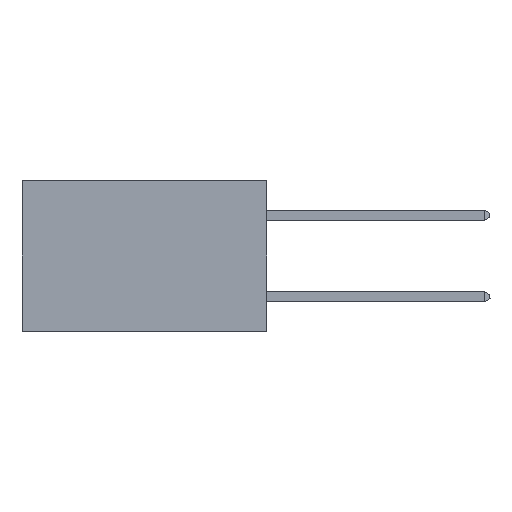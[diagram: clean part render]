
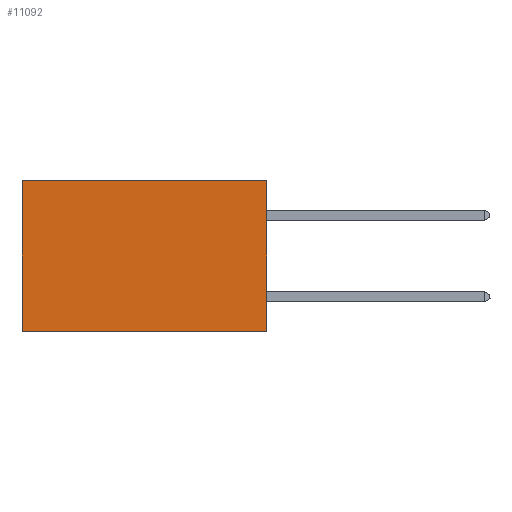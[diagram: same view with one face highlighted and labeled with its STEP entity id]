
A CAD part, left-side view. The second image highlights one B-rep face of the part: STEP entity #11092.
In plain terms, the highlighted planar face has unit normal (-1, 0, 0).
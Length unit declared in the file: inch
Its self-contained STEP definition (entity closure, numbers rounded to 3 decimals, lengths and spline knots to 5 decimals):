
#454 = AXIS2_PLACEMENT_3D ( 'NONE', #13545, #6897, #18457 ) ;
#1673 = ORIENTED_EDGE ( 'NONE', *, *, #16021, .F. ) ;
#1769 = ORIENTED_EDGE ( 'NONE', *, *, #9709, .F. ) ;
#2898 = LINE ( 'NONE', #5772, #15723 ) ;
#3300 = DIRECTION ( 'NONE',  ( 0., 0., -1. ) ) ;
#3677 = VECTOR ( 'NONE', #7392, 39.37008 ) ;
#3735 = EDGE_CURVE ( 'NONE', #11510, #10776, #2898, .T. ) ;
#4346 = EDGE_CURVE ( 'NONE', #15177, #11510, #18508, .T. ) ;
#4684 = CARTESIAN_POINT ( 'NONE',  ( 0.2875, 0., 0. ) ) ;
#5166 = PLANE ( 'NONE',  #454 ) ;
#5332 = VECTOR ( 'NONE', #5885, 39.37008 ) ;
#5772 = CARTESIAN_POINT ( 'NONE',  ( 0.2875, 0.6, 0. ) ) ;
#5885 = DIRECTION ( 'NONE',  ( 0., 1., 0. ) ) ;
#6267 = CARTESIAN_POINT ( 'NONE',  ( 0.2875, 0.6, 0. ) ) ;
#6675 = LINE ( 'NONE', #13383, #15516 ) ;
#6897 = DIRECTION ( 'NONE',  ( 1., 0., 0. ) ) ;
#7115 = ORIENTED_EDGE ( 'NONE', *, *, #3735, .T. ) ;
#7392 = DIRECTION ( 'NONE',  ( 0., 1., 0. ) ) ;
#7498 = DIRECTION ( 'NONE',  ( 0., 0., -1. ) ) ;
#9268 = CARTESIAN_POINT ( 'NONE',  ( 0.2875, 0., -0.37 ) ) ;
#9709 = EDGE_CURVE ( 'NONE', #15177, #10811, #6675, .T. ) ;
#10734 = CARTESIAN_POINT ( 'NONE',  ( 0.2875, 0., 0. ) ) ;
#10776 = VERTEX_POINT ( 'NONE', #12766 ) ;
#10811 = VERTEX_POINT ( 'NONE', #12911 ) ;
#11092 = ADVANCED_FACE ( 'NONE', ( #17744 ), #5166, .F. ) ;
#11510 = VERTEX_POINT ( 'NONE', #6267 ) ;
#11865 = EDGE_LOOP ( 'NONE', ( #7115, #1673, #1769, #18354 ) ) ;
#12766 = CARTESIAN_POINT ( 'NONE',  ( 0.2875, 0.6, -0.37 ) ) ;
#12911 = CARTESIAN_POINT ( 'NONE',  ( 0.2875, 0., -0.37 ) ) ;
#13383 = CARTESIAN_POINT ( 'NONE',  ( 0.2875, 0., 0. ) ) ;
#13545 = CARTESIAN_POINT ( 'NONE',  ( 0.2875, 0., 0. ) ) ;
#14234 = LINE ( 'NONE', #9268, #5332 ) ;
#15177 = VERTEX_POINT ( 'NONE', #4684 ) ;
#15516 = VECTOR ( 'NONE', #3300, 39.37008 ) ;
#15723 = VECTOR ( 'NONE', #7498, 39.37008 ) ;
#16021 = EDGE_CURVE ( 'NONE', #10811, #10776, #14234, .T. ) ;
#17744 = FACE_OUTER_BOUND ( 'NONE', #11865, .T. ) ;
#18354 = ORIENTED_EDGE ( 'NONE', *, *, #4346, .T. ) ;
#18457 = DIRECTION ( 'NONE',  ( 0., 0., -1. ) ) ;
#18508 = LINE ( 'NONE', #10734, #3677 ) ;
